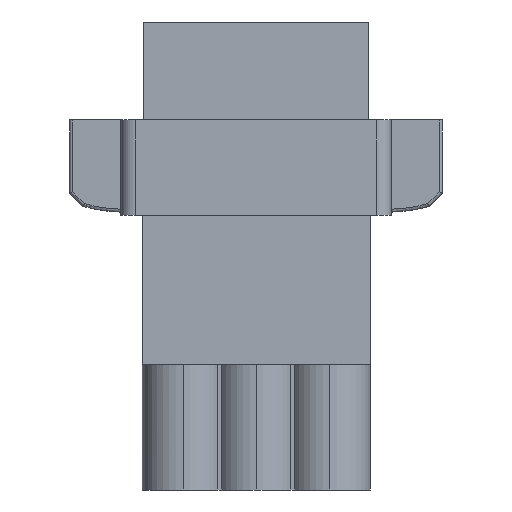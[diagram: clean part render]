
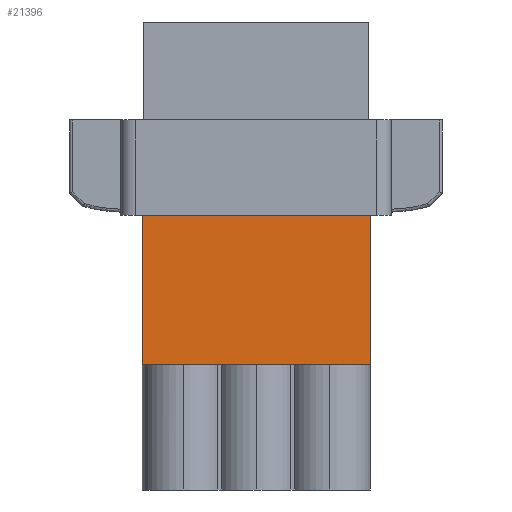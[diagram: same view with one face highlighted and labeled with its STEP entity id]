
A CAD part, front view. The second image highlights one B-rep face of the part: STEP entity #21396.
In plain terms, the highlighted planar face has unit normal (0, -1, 0).
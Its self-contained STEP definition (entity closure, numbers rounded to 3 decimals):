
#191 = VERTEX_POINT ( 'NONE', #1226 ) ;
#641 = CARTESIAN_POINT ( 'NONE',  ( -7.775, -9.275, 0. ) ) ;
#970 = CARTESIAN_POINT ( 'NONE',  ( 0., -9.275, -10.2 ) ) ;
#1187 = DIRECTION ( 'NONE',  ( 1., 0., 0. ) ) ;
#1226 = CARTESIAN_POINT ( 'NONE',  ( -7.775, -9.275, -10.2 ) ) ;
#1695 = ORIENTED_EDGE ( 'NONE', *, *, #1765, .F. ) ;
#1765 = EDGE_CURVE ( 'NONE', #16000, #22475, #4589, .T. ) ;
#2593 = FACE_OUTER_BOUND ( 'NONE', #20944, .T. ) ;
#3990 = VECTOR ( 'NONE', #5746, 1000. ) ;
#4474 = CARTESIAN_POINT ( 'NONE',  ( 0., -9.275, -10.2 ) ) ;
#4589 = LINE ( 'NONE', #15301, #11494 ) ;
#4730 = LINE ( 'NONE', #970, #17889 ) ;
#5326 = EDGE_CURVE ( 'NONE', #191, #16000, #11168, .T. ) ;
#5746 = DIRECTION ( 'NONE',  ( 0., 0., 1. ) ) ;
#7944 = EDGE_CURVE ( 'NONE', #11075, #22475, #11766, .T. ) ;
#8108 = PLANE ( 'NONE',  #16626 ) ;
#8159 = VECTOR ( 'NONE', #13888, 1000. ) ;
#11075 = VERTEX_POINT ( 'NONE', #15540 ) ;
#11168 = LINE ( 'NONE', #16456, #3990 ) ;
#11494 = VECTOR ( 'NONE', #1187, 1000. ) ;
#11642 = DIRECTION ( 'NONE',  ( 0., -1., 0. ) ) ;
#11766 = LINE ( 'NONE', #15421, #8159 ) ;
#13156 = ORIENTED_EDGE ( 'NONE', *, *, #14771, .T. ) ;
#13305 = DIRECTION ( 'NONE',  ( 1., 0., 0. ) ) ;
#13888 = DIRECTION ( 'NONE',  ( 0., 0., 1. ) ) ;
#14771 = EDGE_CURVE ( 'NONE', #191, #11075, #4730, .T. ) ;
#15301 = CARTESIAN_POINT ( 'NONE',  ( 0., -9.275, 0. ) ) ;
#15421 = CARTESIAN_POINT ( 'NONE',  ( 7.825, -9.275, -10.2 ) ) ;
#15540 = CARTESIAN_POINT ( 'NONE',  ( 7.825, -9.275, -10.2 ) ) ;
#16000 = VERTEX_POINT ( 'NONE', #641 ) ;
#16456 = CARTESIAN_POINT ( 'NONE',  ( -7.775, -9.275, -10.2 ) ) ;
#16626 = AXIS2_PLACEMENT_3D ( 'NONE', #4474, #11642, #16698 ) ;
#16698 = DIRECTION ( 'NONE',  ( 0., 0., -1. ) ) ;
#17318 = ORIENTED_EDGE ( 'NONE', *, *, #7944, .T. ) ;
#17889 = VECTOR ( 'NONE', #13305, 1000. ) ;
#18237 = CARTESIAN_POINT ( 'NONE',  ( 7.825, -9.275, 0. ) ) ;
#20944 = EDGE_LOOP ( 'NONE', ( #1695, #22441, #13156, #17318 ) ) ;
#21396 = ADVANCED_FACE ( 'NONE', ( #2593 ), #8108, .T. ) ;
#22441 = ORIENTED_EDGE ( 'NONE', *, *, #5326, .F. ) ;
#22475 = VERTEX_POINT ( 'NONE', #18237 ) ;
